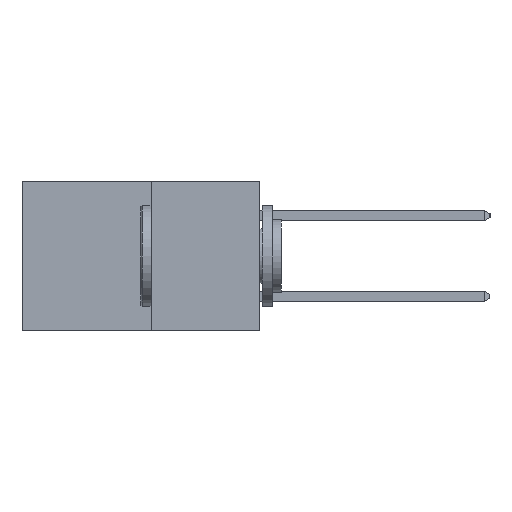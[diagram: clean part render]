
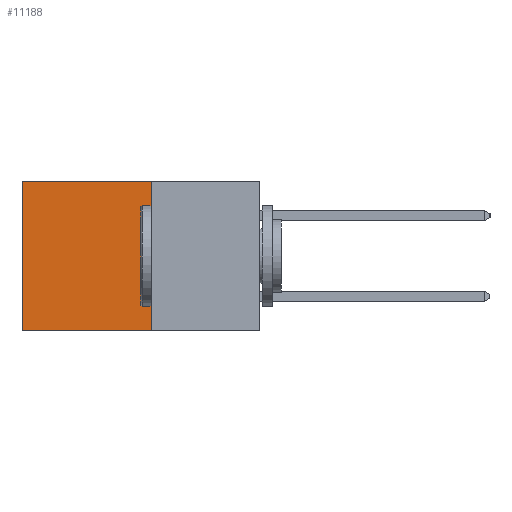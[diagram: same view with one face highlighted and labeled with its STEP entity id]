
A CAD part, left-side view. The second image highlights one B-rep face of the part: STEP entity #11188.
In plain terms, the highlighted planar face has unit normal (-1, 0, 0).
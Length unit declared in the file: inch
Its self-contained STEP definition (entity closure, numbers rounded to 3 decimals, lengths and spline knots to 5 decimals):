
#294 = EDGE_CURVE ( 'NONE', #4159, #8584, #10119, .T. ) ;
#333 = CARTESIAN_POINT ( 'NONE',  ( 0.277, 0.27, -0.37 ) ) ;
#372 = LINE ( 'NONE', #11132, #6403 ) ;
#480 = VECTOR ( 'NONE', #13183, 39.37008 ) ;
#882 = DIRECTION ( 'NONE',  ( 0., 0., -1. ) ) ;
#1752 = VECTOR ( 'NONE', #9441, 39.37008 ) ;
#1810 = EDGE_LOOP ( 'NONE', ( #12923, #2107, #6448, #12211 ) ) ;
#1820 = CARTESIAN_POINT ( 'NONE',  ( 0.277, 0.27, -0.37 ) ) ;
#2107 = ORIENTED_EDGE ( 'NONE', *, *, #10137, .F. ) ;
#4159 = VERTEX_POINT ( 'NONE', #6467 ) ;
#4402 = CARTESIAN_POINT ( 'NONE',  ( 0.277, 0.27, -0.37 ) ) ;
#4673 = EDGE_CURVE ( 'NONE', #7736, #5861, #5348, .T. ) ;
#5333 = FACE_OUTER_BOUND ( 'NONE', #1810, .T. ) ;
#5348 = LINE ( 'NONE', #1820, #1752 ) ;
#5861 = VERTEX_POINT ( 'NONE', #10586 ) ;
#6403 = VECTOR ( 'NONE', #10536, 39.37008 ) ;
#6448 = ORIENTED_EDGE ( 'NONE', *, *, #4673, .F. ) ;
#6467 = CARTESIAN_POINT ( 'NONE',  ( 0.277, 0.59, 0. ) ) ;
#7572 = DIRECTION ( 'NONE',  ( 0., 1., 0. ) ) ;
#7736 = VERTEX_POINT ( 'NONE', #12481 ) ;
#7822 = EDGE_CURVE ( 'NONE', #7736, #4159, #372, .T. ) ;
#8160 = DIRECTION ( 'NONE',  ( 1., 0., 0. ) ) ;
#8584 = VERTEX_POINT ( 'NONE', #11748 ) ;
#9441 = DIRECTION ( 'NONE',  ( 0., 0., -1. ) ) ;
#10119 = LINE ( 'NONE', #12525, #480 ) ;
#10137 = EDGE_CURVE ( 'NONE', #5861, #8584, #13165, .T. ) ;
#10536 = DIRECTION ( 'NONE',  ( 0., 1., 0. ) ) ;
#10586 = CARTESIAN_POINT ( 'NONE',  ( 0.277, 0.27, -0.37 ) ) ;
#11132 = CARTESIAN_POINT ( 'NONE',  ( 0.277, 0.27, 0. ) ) ;
#11188 = ADVANCED_FACE ( 'NONE', ( #5333 ), #15011, .F. ) ;
#11748 = CARTESIAN_POINT ( 'NONE',  ( 0.277, 0.59, -0.37 ) ) ;
#11802 = AXIS2_PLACEMENT_3D ( 'NONE', #4402, #8160, #882 ) ;
#12211 = ORIENTED_EDGE ( 'NONE', *, *, #7822, .T. ) ;
#12481 = CARTESIAN_POINT ( 'NONE',  ( 0.277, 0.27, 0. ) ) ;
#12525 = CARTESIAN_POINT ( 'NONE',  ( 0.277, 0.59, -0.37 ) ) ;
#12813 = VECTOR ( 'NONE', #7572, 39.37008 ) ;
#12923 = ORIENTED_EDGE ( 'NONE', *, *, #294, .T. ) ;
#13165 = LINE ( 'NONE', #333, #12813 ) ;
#13183 = DIRECTION ( 'NONE',  ( 0., 0., -1. ) ) ;
#15011 = PLANE ( 'NONE',  #11802 ) ;
